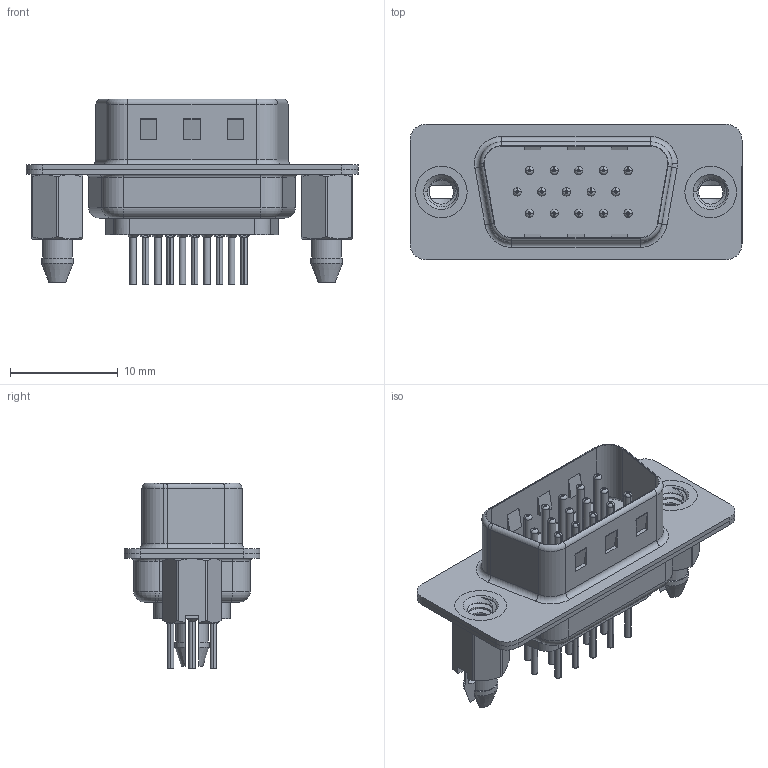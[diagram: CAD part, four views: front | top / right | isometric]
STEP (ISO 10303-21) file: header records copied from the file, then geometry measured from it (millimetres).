
FILE_DESCRIPTION (( 'STEP AP203' ), '1' );
FILE_NAME ('637-015-630-046.STEP', '2020-07-17T23:38:15', ( '' ), ( '' ), 'SwSTEP 2.0', 'SolidWorks 2020', '' );
FILE_SCHEMA (( 'CONFIG_CONTROL_DESIGN' ));
Length unit declared in the file: millimetre
Products named in the file (8): 637 Shell Rear_15 Contacts; 637-015-630-046; 637 Shell Front_15 Contacts; 637 Contact Row 2_30; 637 4-40 Threaded Boardlock_LP; 637 Contact Row 1_30; 637 Housing_15 Contacts; 637 Contact Row 3_30
Assembly tree (20 placements, depth 2):
  637-015-630-046
    637 Housing_15 Contacts
    637 Shell Front_15 Contacts
    637 Shell Rear_15 Contacts
    637 Contact Row 1_30  x5
    637 Contact Row 2_30  x5
    637 Contact Row 3_30  x5
    637 4-40 Threaded Boardlock_LP  x2
Bounding box: 30.8 x 12.6 x 17.25 mm (x, y, z)
Volume: 1429.5 mm3; surface area: 4932.6 mm2
Topology: 20 solids, 20 shells, 1878 faces, 4964 edges, 3075 vertices
Faces by surface type: cylinder 716, plane 499, torus 485, cone 172, bspline 6
Entity records: 24471 total; most frequent: CARTESIAN_POINT 5880, DIRECTION 3882, ORIENTED_EDGE 3558, EDGE_CURVE 1779, AXIS2_PLACEMENT_3D 1571, VERTEX_POINT 1127, CIRCLE 847, EDGE_LOOP 798
